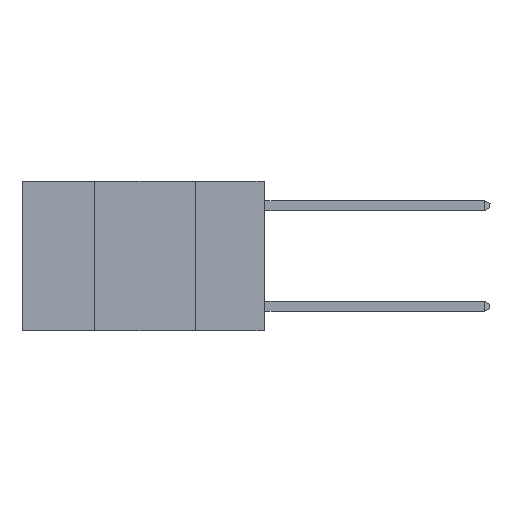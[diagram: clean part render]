
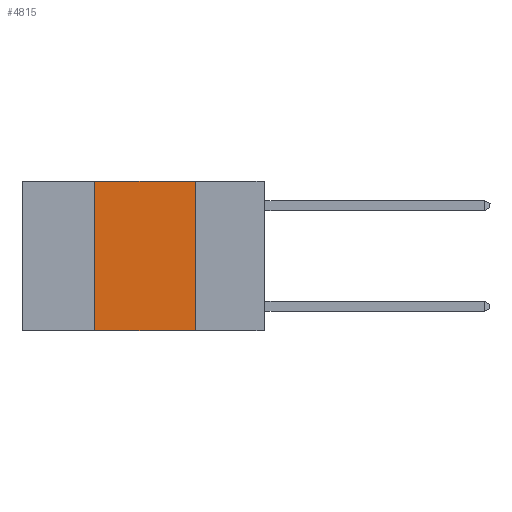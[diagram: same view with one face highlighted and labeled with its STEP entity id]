
A CAD part, left-side view. The second image highlights one B-rep face of the part: STEP entity #4815.
In plain terms, the highlighted planar face has unit normal (-1, 0, 0).
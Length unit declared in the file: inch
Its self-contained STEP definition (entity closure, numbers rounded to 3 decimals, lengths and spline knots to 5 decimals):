
#359 = VERTEX_POINT ( 'NONE', #8761 ) ;
#421 = ORIENTED_EDGE ( 'NONE', *, *, #6548, .T. ) ;
#527 = DIRECTION ( 'NONE',  ( 0., 0., 1. ) ) ;
#1369 = CARTESIAN_POINT ( 'NONE',  ( 0., 0.6, -0.37 ) ) ;
#2065 = FACE_OUTER_BOUND ( 'NONE', #5125, .T. ) ;
#2852 = DIRECTION ( 'NONE',  ( 0., 0., -1. ) ) ;
#3266 = VECTOR ( 'NONE', #527, 39.37008 ) ;
#3303 = VERTEX_POINT ( 'NONE', #3885 ) ;
#3573 = CARTESIAN_POINT ( 'NONE',  ( 0., 0.6, 0. ) ) ;
#3779 = LINE ( 'NONE', #7546, #7910 ) ;
#3885 = CARTESIAN_POINT ( 'NONE',  ( 0., 0.42, -0.37 ) ) ;
#4192 = CARTESIAN_POINT ( 'NONE',  ( 0., 0.6, 0. ) ) ;
#4505 = CARTESIAN_POINT ( 'NONE',  ( 0., 0.42, 0. ) ) ;
#4815 = ADVANCED_FACE ( 'NONE', ( #2065 ), #6433, .F. ) ;
#4922 = EDGE_CURVE ( 'NONE', #359, #8525, #3779, .T. ) ;
#4927 = ORIENTED_EDGE ( 'NONE', *, *, #4922, .F. ) ;
#5125 = EDGE_LOOP ( 'NONE', ( #4927, #7553, #7338, #421 ) ) ;
#5147 = LINE ( 'NONE', #1369, #9030 ) ;
#5985 = DIRECTION ( 'NONE',  ( 0., 0., -1. ) ) ;
#6433 = PLANE ( 'NONE',  #8531 ) ;
#6491 = LINE ( 'NONE', #8037, #3266 ) ;
#6548 = EDGE_CURVE ( 'NONE', #3303, #8525, #5147, .T. ) ;
#6569 = DIRECTION ( 'NONE',  ( 0., -1., 0. ) ) ;
#6573 = DIRECTION ( 'NONE',  ( 1., 0., 0. ) ) ;
#7173 = DIRECTION ( 'NONE',  ( 0., -1., 0. ) ) ;
#7230 = VERTEX_POINT ( 'NONE', #4505 ) ;
#7338 = ORIENTED_EDGE ( 'NONE', *, *, #7523, .F. ) ;
#7523 = EDGE_CURVE ( 'NONE', #3303, #7230, #6491, .T. ) ;
#7546 = CARTESIAN_POINT ( 'NONE',  ( 0., 0.17, 0. ) ) ;
#7553 = ORIENTED_EDGE ( 'NONE', *, *, #9220, .F. ) ;
#7683 = CARTESIAN_POINT ( 'NONE',  ( 0., 0.17, -0.37 ) ) ;
#7891 = LINE ( 'NONE', #4192, #8913 ) ;
#7910 = VECTOR ( 'NONE', #5985, 39.37008 ) ;
#8037 = CARTESIAN_POINT ( 'NONE',  ( 0., 0.42, 0. ) ) ;
#8525 = VERTEX_POINT ( 'NONE', #7683 ) ;
#8531 = AXIS2_PLACEMENT_3D ( 'NONE', #3573, #6573, #2852 ) ;
#8761 = CARTESIAN_POINT ( 'NONE',  ( 0., 0.17, 0. ) ) ;
#8913 = VECTOR ( 'NONE', #7173, 39.37008 ) ;
#9030 = VECTOR ( 'NONE', #6569, 39.37008 ) ;
#9220 = EDGE_CURVE ( 'NONE', #7230, #359, #7891, .T. ) ;
